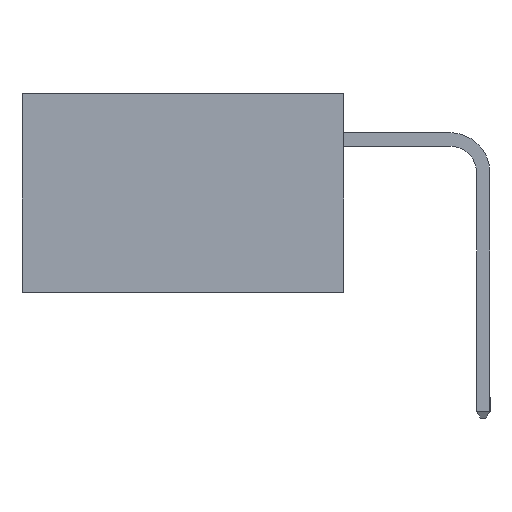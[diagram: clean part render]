
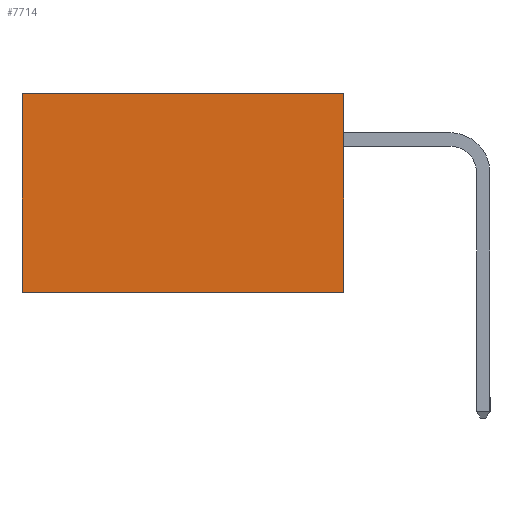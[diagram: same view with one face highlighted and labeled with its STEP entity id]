
A CAD part, left-side view. The second image highlights one B-rep face of the part: STEP entity #7714.
In plain terms, the highlighted planar face has unit normal (-1, 0, 0).
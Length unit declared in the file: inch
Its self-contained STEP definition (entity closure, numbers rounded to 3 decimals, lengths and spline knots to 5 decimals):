
#282 = CARTESIAN_POINT ( 'NONE',  ( 0.2615, 0., -0.37 ) ) ;
#852 = DIRECTION ( 'NONE',  ( 0., 0., -1. ) ) ;
#916 = CARTESIAN_POINT ( 'NONE',  ( 0.2615, 0., -0.37 ) ) ;
#1067 = DIRECTION ( 'NONE',  ( 0., 0., -1. ) ) ;
#1094 = DIRECTION ( 'NONE',  ( 1., 0., 0. ) ) ;
#1154 = PLANE ( 'NONE',  #11207 ) ;
#1515 = CARTESIAN_POINT ( 'NONE',  ( 0.2615, 0., -0.37 ) ) ;
#3019 = LINE ( 'NONE', #916, #19455 ) ;
#3879 = EDGE_LOOP ( 'NONE', ( #17168, #14977, #19973, #17728 ) ) ;
#4179 = DIRECTION ( 'NONE',  ( 0., 1., 0. ) ) ;
#4255 = LINE ( 'NONE', #12634, #16554 ) ;
#4678 = VERTEX_POINT ( 'NONE', #16365 ) ;
#4976 = CARTESIAN_POINT ( 'NONE',  ( 0.2615, 0., 0. ) ) ;
#5182 = CARTESIAN_POINT ( 'NONE',  ( 0.2615, 0.6, 0. ) ) ;
#7714 = ADVANCED_FACE ( 'NONE', ( #11828 ), #1154, .F. ) ;
#7729 = EDGE_CURVE ( 'NONE', #13175, #4678, #3019, .T. ) ;
#8327 = EDGE_CURVE ( 'NONE', #4678, #19350, #20554, .T. ) ;
#11207 = AXIS2_PLACEMENT_3D ( 'NONE', #1515, #1094, #1067 ) ;
#11828 = FACE_OUTER_BOUND ( 'NONE', #3879, .T. ) ;
#11935 = EDGE_CURVE ( 'NONE', #20316, #19350, #4255, .T. ) ;
#12169 = CARTESIAN_POINT ( 'NONE',  ( 0.2615, 0., 0. ) ) ;
#12422 = CARTESIAN_POINT ( 'NONE',  ( 0.2615, 0.6, -0.37 ) ) ;
#12597 = DIRECTION ( 'NONE',  ( 0., 0., -1. ) ) ;
#12634 = CARTESIAN_POINT ( 'NONE',  ( 0.2615, 0.6, -0.37 ) ) ;
#13175 = VERTEX_POINT ( 'NONE', #12169 ) ;
#13818 = VECTOR ( 'NONE', #4179, 39.37008 ) ;
#14710 = EDGE_CURVE ( 'NONE', #13175, #20316, #18336, .T. ) ;
#14977 = ORIENTED_EDGE ( 'NONE', *, *, #8327, .F. ) ;
#16115 = VECTOR ( 'NONE', #20663, 39.37008 ) ;
#16365 = CARTESIAN_POINT ( 'NONE',  ( 0.2615, 0., -0.37 ) ) ;
#16554 = VECTOR ( 'NONE', #12597, 39.37008 ) ;
#17168 = ORIENTED_EDGE ( 'NONE', *, *, #11935, .T. ) ;
#17728 = ORIENTED_EDGE ( 'NONE', *, *, #14710, .T. ) ;
#18336 = LINE ( 'NONE', #4976, #13818 ) ;
#19350 = VERTEX_POINT ( 'NONE', #12422 ) ;
#19455 = VECTOR ( 'NONE', #852, 39.37008 ) ;
#19973 = ORIENTED_EDGE ( 'NONE', *, *, #7729, .F. ) ;
#20316 = VERTEX_POINT ( 'NONE', #5182 ) ;
#20554 = LINE ( 'NONE', #282, #16115 ) ;
#20663 = DIRECTION ( 'NONE',  ( 0., 1., 0. ) ) ;
